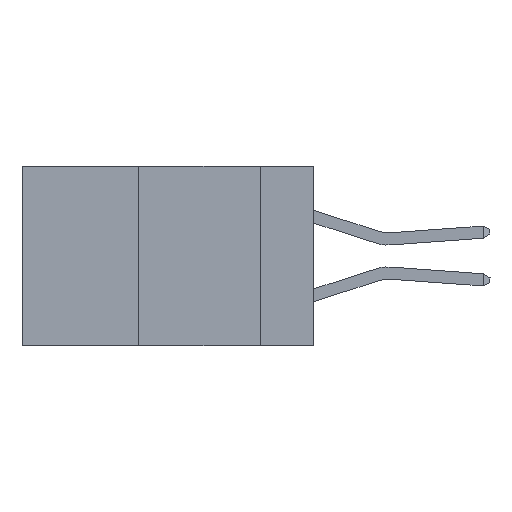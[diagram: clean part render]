
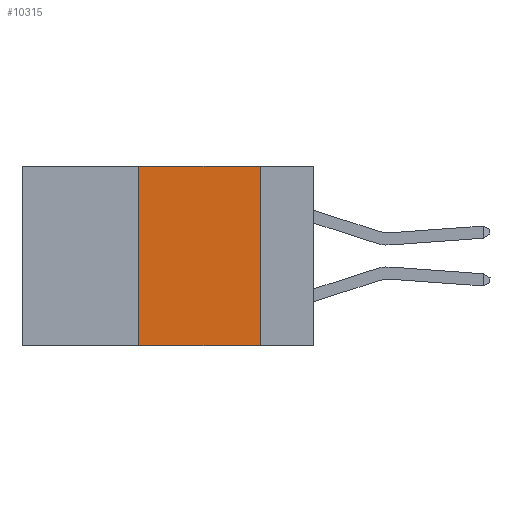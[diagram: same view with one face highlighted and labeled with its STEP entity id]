
A CAD part, left-side view. The second image highlights one B-rep face of the part: STEP entity #10315.
In plain terms, the highlighted planar face has unit normal (-1, 0, 0).
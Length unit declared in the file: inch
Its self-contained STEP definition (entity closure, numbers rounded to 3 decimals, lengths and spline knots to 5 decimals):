
#305 = AXIS2_PLACEMENT_3D ( 'NONE', #5421, #5329, #26013 ) ;
#2430 = CARTESIAN_POINT ( 'NONE',  ( 0., 0.11, 0. ) ) ;
#3406 = LINE ( 'NONE', #11219, #8889 ) ;
#3732 = EDGE_LOOP ( 'NONE', ( #9902, #19052, #9009, #11739 ) ) ;
#4674 = VERTEX_POINT ( 'NONE', #16334 ) ;
#5329 = DIRECTION ( 'NONE',  ( 1., 0., 0. ) ) ;
#5421 = CARTESIAN_POINT ( 'NONE',  ( 0., 0.6, 0. ) ) ;
#5671 = VECTOR ( 'NONE', #14002, 39.37008 ) ;
#6884 = LINE ( 'NONE', #24063, #11952 ) ;
#7653 = VECTOR ( 'NONE', #21940, 39.37008 ) ;
#8889 = VECTOR ( 'NONE', #24684, 39.37008 ) ;
#9009 = ORIENTED_EDGE ( 'NONE', *, *, #24238, .F. ) ;
#9332 = LINE ( 'NONE', #20685, #5671 ) ;
#9432 = CARTESIAN_POINT ( 'NONE',  ( 0., 0.36, 0. ) ) ;
#9902 = ORIENTED_EDGE ( 'NONE', *, *, #27653, .F. ) ;
#10315 = ADVANCED_FACE ( 'NONE', ( #10706 ), #19120, .F. ) ;
#10706 = FACE_OUTER_BOUND ( 'NONE', #3732, .T. ) ;
#10914 = LINE ( 'NONE', #15000, #7653 ) ;
#11219 = CARTESIAN_POINT ( 'NONE',  ( 0., 0.6, 0. ) ) ;
#11739 = ORIENTED_EDGE ( 'NONE', *, *, #19908, .T. ) ;
#11952 = VECTOR ( 'NONE', #24475, 39.37008 ) ;
#14002 = DIRECTION ( 'NONE',  ( 0., -1., 0. ) ) ;
#15000 = CARTESIAN_POINT ( 'NONE',  ( 0., 0.36, 0. ) ) ;
#15906 = VERTEX_POINT ( 'NONE', #2430 ) ;
#16334 = CARTESIAN_POINT ( 'NONE',  ( 0., 0.11, -0.37 ) ) ;
#19052 = ORIENTED_EDGE ( 'NONE', *, *, #27706, .F. ) ;
#19120 = PLANE ( 'NONE',  #305 ) ;
#19891 = VERTEX_POINT ( 'NONE', #9432 ) ;
#19908 = EDGE_CURVE ( 'NONE', #23794, #4674, #9332, .T. ) ;
#20685 = CARTESIAN_POINT ( 'NONE',  ( 0., 0.6, -0.37 ) ) ;
#21940 = DIRECTION ( 'NONE',  ( 0., 0., 1. ) ) ;
#23794 = VERTEX_POINT ( 'NONE', #29002 ) ;
#24063 = CARTESIAN_POINT ( 'NONE',  ( 0., 0.11, 0. ) ) ;
#24238 = EDGE_CURVE ( 'NONE', #23794, #19891, #10914, .T. ) ;
#24475 = DIRECTION ( 'NONE',  ( 0., 0., -1. ) ) ;
#24684 = DIRECTION ( 'NONE',  ( 0., -1., 0. ) ) ;
#26013 = DIRECTION ( 'NONE',  ( 0., 0., -1. ) ) ;
#27653 = EDGE_CURVE ( 'NONE', #15906, #4674, #6884, .T. ) ;
#27706 = EDGE_CURVE ( 'NONE', #19891, #15906, #3406, .T. ) ;
#29002 = CARTESIAN_POINT ( 'NONE',  ( 0., 0.36, -0.37 ) ) ;
